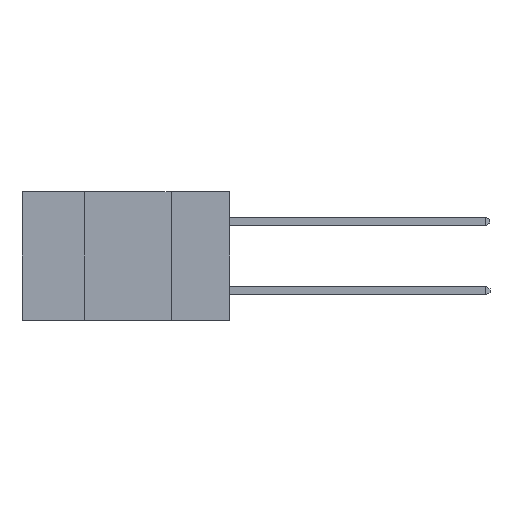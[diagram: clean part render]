
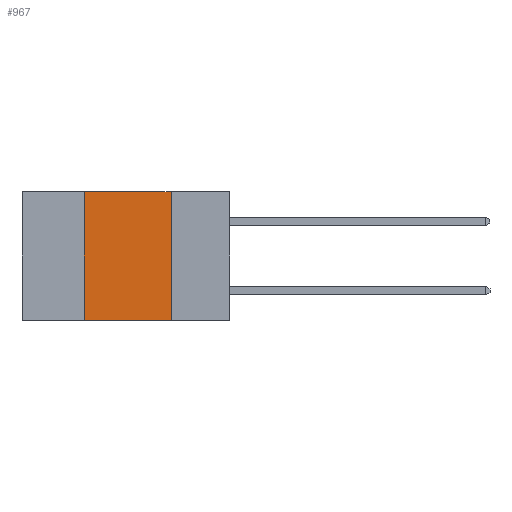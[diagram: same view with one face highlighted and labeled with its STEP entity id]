
A CAD part, left-side view. The second image highlights one B-rep face of the part: STEP entity #967.
In plain terms, the highlighted planar face has unit normal (-1, 0, 0).
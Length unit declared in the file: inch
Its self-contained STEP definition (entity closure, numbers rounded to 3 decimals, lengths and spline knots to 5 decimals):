
#77 = EDGE_CURVE ( 'NONE', #6608, #4131, #7979, .T. ) ;
#117 = VECTOR ( 'NONE', #1002, 39.37008 ) ;
#165 = CARTESIAN_POINT ( 'NONE',  ( 0., 0.17, -0.37 ) ) ;
#204 = CARTESIAN_POINT ( 'NONE',  ( 0., 0.6, 0. ) ) ;
#773 = VECTOR ( 'NONE', #7039, 39.37008 ) ;
#825 = DIRECTION ( 'NONE',  ( 1., 0., 0. ) ) ;
#868 = CARTESIAN_POINT ( 'NONE',  ( 0., 0.42, 0. ) ) ;
#917 = PLANE ( 'NONE',  #8290 ) ;
#967 = ADVANCED_FACE ( 'NONE', ( #6251 ), #917, .F. ) ;
#1002 = DIRECTION ( 'NONE',  ( 0., 0., -1. ) ) ;
#1034 = DIRECTION ( 'NONE',  ( 0., -1., 0. ) ) ;
#1168 = VERTEX_POINT ( 'NONE', #868 ) ;
#1200 = VECTOR ( 'NONE', #4331, 39.37008 ) ;
#1224 = EDGE_LOOP ( 'NONE', ( #4761, #4790, #7162, #7111 ) ) ;
#1228 = CARTESIAN_POINT ( 'NONE',  ( 0., 0.6, 0. ) ) ;
#1638 = CARTESIAN_POINT ( 'NONE',  ( 0., 0.42, -0.37 ) ) ;
#2255 = DIRECTION ( 'NONE',  ( 0., 0., -1. ) ) ;
#2654 = LINE ( 'NONE', #6395, #773 ) ;
#2968 = CARTESIAN_POINT ( 'NONE',  ( 0., 0.6, -0.37 ) ) ;
#4131 = VERTEX_POINT ( 'NONE', #5882 ) ;
#4331 = DIRECTION ( 'NONE',  ( 0., -1., 0. ) ) ;
#4761 = ORIENTED_EDGE ( 'NONE', *, *, #7559, .F. ) ;
#4790 = ORIENTED_EDGE ( 'NONE', *, *, #7582, .F. ) ;
#5423 = LINE ( 'NONE', #204, #8603 ) ;
#5882 = CARTESIAN_POINT ( 'NONE',  ( 0., 0.17, -0.37 ) ) ;
#6251 = FACE_OUTER_BOUND ( 'NONE', #1224, .T. ) ;
#6395 = CARTESIAN_POINT ( 'NONE',  ( 0., 0.42, -0.37 ) ) ;
#6608 = VERTEX_POINT ( 'NONE', #1638 ) ;
#6620 = VERTEX_POINT ( 'NONE', #7538 ) ;
#7039 = DIRECTION ( 'NONE',  ( 0., 0., 1. ) ) ;
#7111 = ORIENTED_EDGE ( 'NONE', *, *, #77, .T. ) ;
#7162 = ORIENTED_EDGE ( 'NONE', *, *, #8402, .F. ) ;
#7329 = LINE ( 'NONE', #165, #117 ) ;
#7538 = CARTESIAN_POINT ( 'NONE',  ( 0., 0.17, 0. ) ) ;
#7559 = EDGE_CURVE ( 'NONE', #6620, #4131, #7329, .T. ) ;
#7582 = EDGE_CURVE ( 'NONE', #1168, #6620, #5423, .T. ) ;
#7979 = LINE ( 'NONE', #2968, #1200 ) ;
#8290 = AXIS2_PLACEMENT_3D ( 'NONE', #1228, #825, #2255 ) ;
#8402 = EDGE_CURVE ( 'NONE', #6608, #1168, #2654, .T. ) ;
#8603 = VECTOR ( 'NONE', #1034, 39.37008 ) ;
